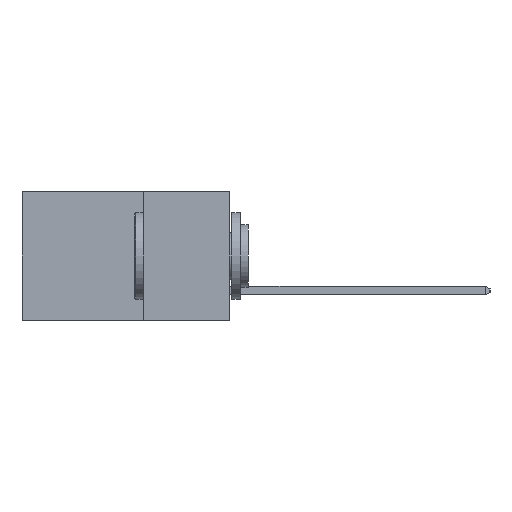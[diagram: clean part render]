
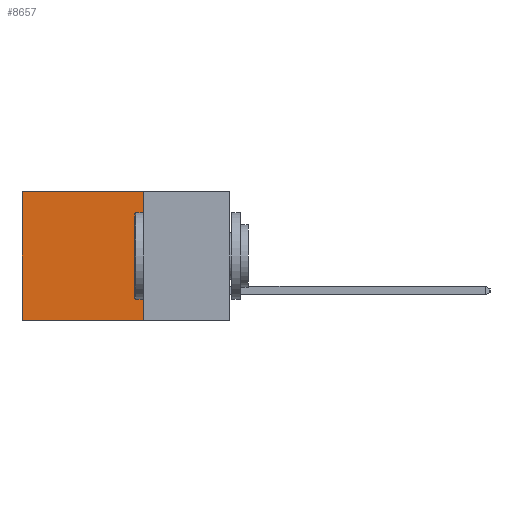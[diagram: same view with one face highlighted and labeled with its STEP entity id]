
A CAD part, left-side view. The second image highlights one B-rep face of the part: STEP entity #8657.
In plain terms, the highlighted planar face has unit normal (-1, 0, 0).
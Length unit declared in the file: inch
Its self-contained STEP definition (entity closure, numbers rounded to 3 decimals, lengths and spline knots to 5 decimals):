
#906 = ORIENTED_EDGE ( 'NONE', *, *, #4631, .F. ) ;
#1108 = ORIENTED_EDGE ( 'NONE', *, *, #1540, .F. ) ;
#1120 = ORIENTED_EDGE ( 'NONE', *, *, #9658, .T. ) ;
#1540 = EDGE_CURVE ( 'NONE', #8212, #9346, #5165, .T. ) ;
#1709 = CARTESIAN_POINT ( 'NONE',  ( 0.298, 0.25, 0. ) ) ;
#1915 = LINE ( 'NONE', #1709, #6689 ) ;
#2126 = VECTOR ( 'NONE', #5804, 39.37008 ) ;
#2583 = CARTESIAN_POINT ( 'NONE',  ( 0.298, 0.25, 0. ) ) ;
#2633 = DIRECTION ( 'NONE',  ( 0., 0., -1. ) ) ;
#2744 = VERTEX_POINT ( 'NONE', #2583 ) ;
#3182 = VERTEX_POINT ( 'NONE', #9746 ) ;
#4301 = CARTESIAN_POINT ( 'NONE',  ( 0.298, 0.25, -0.37 ) ) ;
#4631 = EDGE_CURVE ( 'NONE', #2744, #8212, #12057, .T. ) ;
#4749 = CARTESIAN_POINT ( 'NONE',  ( 0.298, 0.25, -0.37 ) ) ;
#5165 = LINE ( 'NONE', #4749, #2126 ) ;
#5804 = DIRECTION ( 'NONE',  ( 0., 1., 0. ) ) ;
#6237 = CARTESIAN_POINT ( 'NONE',  ( 0.298, 0.25, 0. ) ) ;
#6540 = VECTOR ( 'NONE', #12172, 39.37008 ) ;
#6689 = VECTOR ( 'NONE', #9990, 39.37008 ) ;
#6914 = CARTESIAN_POINT ( 'NONE',  ( 0.298, 0.25, 0. ) ) ;
#6971 = DIRECTION ( 'NONE',  ( 0., 0., -1. ) ) ;
#7461 = EDGE_LOOP ( 'NONE', ( #1120, #1108, #906, #8947 ) ) ;
#8212 = VERTEX_POINT ( 'NONE', #4301 ) ;
#8657 = ADVANCED_FACE ( 'NONE', ( #10771 ), #12146, .F. ) ;
#8735 = CARTESIAN_POINT ( 'NONE',  ( 0.298, 0.6, 0. ) ) ;
#8947 = ORIENTED_EDGE ( 'NONE', *, *, #11796, .T. ) ;
#9346 = VERTEX_POINT ( 'NONE', #11031 ) ;
#9658 = EDGE_CURVE ( 'NONE', #3182, #9346, #9788, .T. ) ;
#9746 = CARTESIAN_POINT ( 'NONE',  ( 0.298, 0.6, 0. ) ) ;
#9788 = LINE ( 'NONE', #8735, #12458 ) ;
#9990 = DIRECTION ( 'NONE',  ( 0., 1., 0. ) ) ;
#10771 = FACE_OUTER_BOUND ( 'NONE', #7461, .T. ) ;
#11031 = CARTESIAN_POINT ( 'NONE',  ( 0.298, 0.6, -0.37 ) ) ;
#11614 = AXIS2_PLACEMENT_3D ( 'NONE', #6914, #13126, #6971 ) ;
#11796 = EDGE_CURVE ( 'NONE', #2744, #3182, #1915, .T. ) ;
#12057 = LINE ( 'NONE', #6237, #6540 ) ;
#12146 = PLANE ( 'NONE',  #11614 ) ;
#12172 = DIRECTION ( 'NONE',  ( 0., 0., -1. ) ) ;
#12458 = VECTOR ( 'NONE', #2633, 39.37008 ) ;
#13126 = DIRECTION ( 'NONE',  ( 1., 0., 0. ) ) ;
